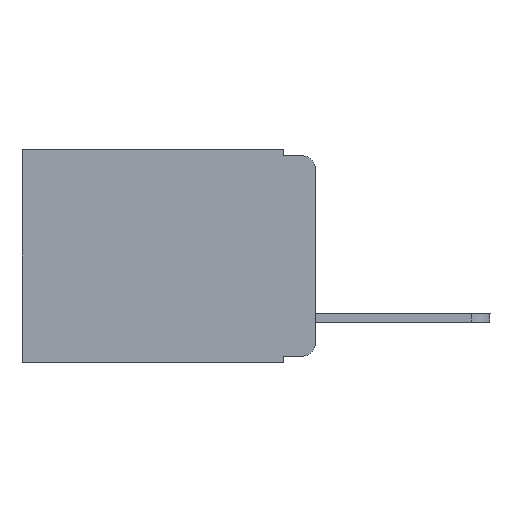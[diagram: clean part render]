
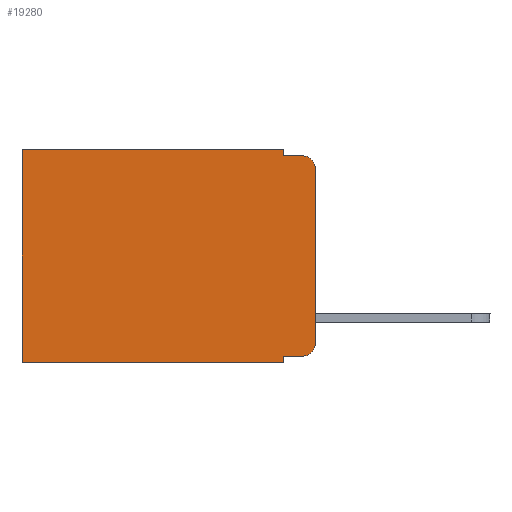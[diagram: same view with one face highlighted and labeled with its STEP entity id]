
A CAD part, left-side view. The second image highlights one B-rep face of the part: STEP entity #19280.
In plain terms, the highlighted planar face has unit normal (-1, 0, 0).
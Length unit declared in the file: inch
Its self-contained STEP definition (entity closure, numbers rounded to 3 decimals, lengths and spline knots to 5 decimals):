
#99 = VERTEX_POINT ( 'NONE', #5547 ) ;
#451 = CARTESIAN_POINT ( 'NONE',  ( 0.298, 0., 0. ) ) ;
#565 = DIRECTION ( 'NONE',  ( 0., 1., 0. ) ) ;
#789 = VERTEX_POINT ( 'NONE', #3210 ) ;
#1083 = VECTOR ( 'NONE', #5646, 39.37008 ) ;
#1096 = EDGE_CURVE ( 'NONE', #4963, #13632, #19596, .T. ) ;
#1431 = DIRECTION ( 'NONE',  ( 0., 0., -1. ) ) ;
#1482 = CARTESIAN_POINT ( 'NONE',  ( 0.298, 0.051, 0. ) ) ;
#1546 = PLANE ( 'NONE',  #18223 ) ;
#1624 = DIRECTION ( 'NONE',  ( 0., -1., 0. ) ) ;
#1875 = LINE ( 'NONE', #4103, #8279 ) ;
#1983 = ORIENTED_EDGE ( 'NONE', *, *, #15755, .T. ) ;
#2217 = EDGE_LOOP ( 'NONE', ( #11682, #13311, #18318, #12543, #4443, #16478, #6858, #9984, #10487, #1983 ) ) ;
#2533 = EDGE_CURVE ( 'NONE', #17612, #16047, #9422, .T. ) ;
#2595 = CARTESIAN_POINT ( 'NONE',  ( 0.298, 0.02, -0.313 ) ) ;
#2623 = EDGE_CURVE ( 'NONE', #6343, #99, #20239, .T. ) ;
#2720 = CARTESIAN_POINT ( 'NONE',  ( 0.298, 0.051, -0.343 ) ) ;
#2898 = CARTESIAN_POINT ( 'NONE',  ( 0.298, 0., 0. ) ) ;
#3003 = CARTESIAN_POINT ( 'NONE',  ( 0.298, 0., 0. ) ) ;
#3210 = CARTESIAN_POINT ( 'NONE',  ( 0.298, 0., -0.313 ) ) ;
#3480 = AXIS2_PLACEMENT_3D ( 'NONE', #2595, #12502, #16734 ) ;
#3509 = CARTESIAN_POINT ( 'NONE',  ( 0.298, 0.051, -0.333 ) ) ;
#3679 = DIRECTION ( 'NONE',  ( -1., 0., 0. ) ) ;
#4103 = CARTESIAN_POINT ( 'NONE',  ( 0.298, 0.051, 0. ) ) ;
#4443 = ORIENTED_EDGE ( 'NONE', *, *, #9549, .T. ) ;
#4646 = VECTOR ( 'NONE', #9031, 39.37008 ) ;
#4963 = VERTEX_POINT ( 'NONE', #1482 ) ;
#5259 = VECTOR ( 'NONE', #16214, 39.37008 ) ;
#5389 = VERTEX_POINT ( 'NONE', #2720 ) ;
#5547 = CARTESIAN_POINT ( 'NONE',  ( 0.298, 0.02, -0.01 ) ) ;
#5646 = DIRECTION ( 'NONE',  ( 0., 0., -1. ) ) ;
#5871 = LINE ( 'NONE', #2898, #4646 ) ;
#6343 = VERTEX_POINT ( 'NONE', #11137 ) ;
#6858 = ORIENTED_EDGE ( 'NONE', *, *, #19060, .F. ) ;
#6953 = CARTESIAN_POINT ( 'NONE',  ( 0.298, 0.02, -0.03 ) ) ;
#7077 = LINE ( 'NONE', #17647, #5259 ) ;
#7297 = CARTESIAN_POINT ( 'NONE',  ( 0.298, 0., -0.343 ) ) ;
#7382 = EDGE_CURVE ( 'NONE', #13632, #99, #7077, .T. ) ;
#7485 = CARTESIAN_POINT ( 'NONE',  ( 0.298, 0.051, 0. ) ) ;
#7766 = EDGE_CURVE ( 'NONE', #16389, #8477, #16365, .T. ) ;
#8279 = VECTOR ( 'NONE', #12860, 39.37008 ) ;
#8477 = VERTEX_POINT ( 'NONE', #10482 ) ;
#9031 = DIRECTION ( 'NONE',  ( 0., 0., -1. ) ) ;
#9422 = LINE ( 'NONE', #15700, #11685 ) ;
#9549 = EDGE_CURVE ( 'NONE', #4963, #16389, #17615, .T. ) ;
#9984 = ORIENTED_EDGE ( 'NONE', *, *, #11629, .F. ) ;
#10094 = DIRECTION ( 'NONE',  ( 0., 0., -1. ) ) ;
#10168 = EDGE_CURVE ( 'NONE', #6343, #789, #5871, .T. ) ;
#10482 = CARTESIAN_POINT ( 'NONE',  ( 0.298, 0.473, -0.343 ) ) ;
#10487 = ORIENTED_EDGE ( 'NONE', *, *, #2533, .T. ) ;
#11137 = CARTESIAN_POINT ( 'NONE',  ( 0.298, 0., -0.03 ) ) ;
#11629 = EDGE_CURVE ( 'NONE', #17612, #5389, #1875, .T. ) ;
#11682 = ORIENTED_EDGE ( 'NONE', *, *, #10168, .F. ) ;
#11683 = DIRECTION ( 'NONE',  ( 0., 0., -1. ) ) ;
#11685 = VECTOR ( 'NONE', #1624, 39.37008 ) ;
#12134 = DIRECTION ( 'NONE',  ( 0., 1., 0. ) ) ;
#12502 = DIRECTION ( 'NONE',  ( -1., 0., 0. ) ) ;
#12543 = ORIENTED_EDGE ( 'NONE', *, *, #1096, .F. ) ;
#12860 = DIRECTION ( 'NONE',  ( 0., 0., -1. ) ) ;
#13311 = ORIENTED_EDGE ( 'NONE', *, *, #2623, .T. ) ;
#13632 = VERTEX_POINT ( 'NONE', #13704 ) ;
#13704 = CARTESIAN_POINT ( 'NONE',  ( 0.298, 0.051, -0.01 ) ) ;
#14162 = DIRECTION ( 'NONE',  ( 1., 0., 0. ) ) ;
#14453 = VECTOR ( 'NONE', #565, 39.37008 ) ;
#14940 = VECTOR ( 'NONE', #12134, 39.37008 ) ;
#15407 = FACE_OUTER_BOUND ( 'NONE', #2217, .T. ) ;
#15601 = CIRCLE ( 'NONE', #3480, 0.02 ) ;
#15700 = CARTESIAN_POINT ( 'NONE',  ( 0.298, 0.051, -0.333 ) ) ;
#15755 = EDGE_CURVE ( 'NONE', #16047, #789, #15601, .T. ) ;
#16047 = VERTEX_POINT ( 'NONE', #17999 ) ;
#16214 = DIRECTION ( 'NONE',  ( 0., -1., 0. ) ) ;
#16365 = LINE ( 'NONE', #19436, #16741 ) ;
#16389 = VERTEX_POINT ( 'NONE', #19584 ) ;
#16478 = ORIENTED_EDGE ( 'NONE', *, *, #7766, .T. ) ;
#16734 = DIRECTION ( 'NONE',  ( 0., 0., -1. ) ) ;
#16741 = VECTOR ( 'NONE', #10094, 39.37008 ) ;
#17299 = AXIS2_PLACEMENT_3D ( 'NONE', #6953, #3679, #11683 ) ;
#17612 = VERTEX_POINT ( 'NONE', #3509 ) ;
#17615 = LINE ( 'NONE', #451, #14453 ) ;
#17647 = CARTESIAN_POINT ( 'NONE',  ( 0.298, 0.051, -0.01 ) ) ;
#17964 = LINE ( 'NONE', #7297, #14940 ) ;
#17999 = CARTESIAN_POINT ( 'NONE',  ( 0.298, 0.02, -0.333 ) ) ;
#18223 = AXIS2_PLACEMENT_3D ( 'NONE', #3003, #14162, #1431 ) ;
#18318 = ORIENTED_EDGE ( 'NONE', *, *, #7382, .F. ) ;
#19060 = EDGE_CURVE ( 'NONE', #5389, #8477, #17964, .T. ) ;
#19280 = ADVANCED_FACE ( 'NONE', ( #15407 ), #1546, .F. ) ;
#19436 = CARTESIAN_POINT ( 'NONE',  ( 0.298, 0.473, 0. ) ) ;
#19584 = CARTESIAN_POINT ( 'NONE',  ( 0.298, 0.473, 0. ) ) ;
#19596 = LINE ( 'NONE', #7485, #1083 ) ;
#20239 = CIRCLE ( 'NONE', #17299, 0.02 ) ;
